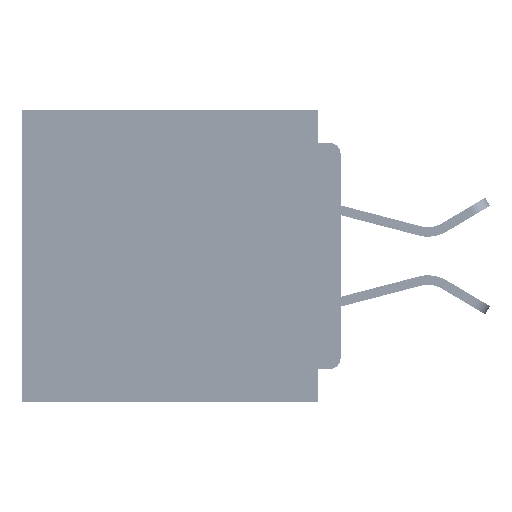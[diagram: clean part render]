
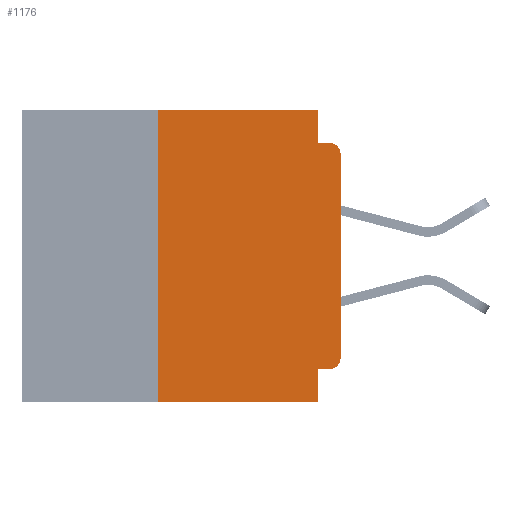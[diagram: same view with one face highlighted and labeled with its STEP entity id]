
A CAD part, left-side view. The second image highlights one B-rep face of the part: STEP entity #1176.
In plain terms, the highlighted planar face has unit normal (-1, 0, 0).
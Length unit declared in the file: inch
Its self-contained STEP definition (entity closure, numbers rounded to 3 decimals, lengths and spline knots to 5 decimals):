
#187 = LINE ( 'NONE', #39883, #10791 ) ;
#500 = CIRCLE ( 'NONE', #19951, 0.015 ) ;
#1176 = ADVANCED_FACE ( 'NONE', ( #3654 ), #41799, .F. ) ;
#2094 = CARTESIAN_POINT ( 'NONE',  ( 0., 0.25, -0.4 ) ) ;
#2684 = CARTESIAN_POINT ( 'NONE',  ( 0., 0.031, 0. ) ) ;
#3654 = FACE_OUTER_BOUND ( 'NONE', #29090, .T. ) ;
#3697 = VECTOR ( 'NONE', #33979, 39.37008 ) ;
#4495 = VECTOR ( 'NONE', #24936, 39.37008 ) ;
#5057 = EDGE_CURVE ( 'NONE', #32782, #6862, #44740, .T. ) ;
#5749 = ORIENTED_EDGE ( 'NONE', *, *, #19472, .T. ) ;
#6282 = DIRECTION ( 'NONE',  ( 0., -1., 0. ) ) ;
#6862 = VERTEX_POINT ( 'NONE', #33075 ) ;
#7333 = ORIENTED_EDGE ( 'NONE', *, *, #5057, .F. ) ;
#7449 = DIRECTION ( 'NONE',  ( -1., 0., 0. ) ) ;
#9366 = EDGE_CURVE ( 'NONE', #20051, #9809, #41578, .T. ) ;
#9436 = LINE ( 'NONE', #13655, #43655 ) ;
#9809 = VERTEX_POINT ( 'NONE', #24323 ) ;
#10075 = CARTESIAN_POINT ( 'NONE',  ( 0., 0.031, -0.355 ) ) ;
#10219 = CIRCLE ( 'NONE', #50465, 0.015 ) ;
#10791 = VECTOR ( 'NONE', #44306, 39.37008 ) ;
#13051 = VERTEX_POINT ( 'NONE', #51636 ) ;
#13473 = VERTEX_POINT ( 'NONE', #10075 ) ;
#13654 = VECTOR ( 'NONE', #21131, 39.37008 ) ;
#13655 = CARTESIAN_POINT ( 'NONE',  ( 0., 0., -0.355 ) ) ;
#14047 = LINE ( 'NONE', #21825, #36419 ) ;
#15650 = LINE ( 'NONE', #2684, #3697 ) ;
#15993 = ORIENTED_EDGE ( 'NONE', *, *, #42915, .T. ) ;
#16497 = CARTESIAN_POINT ( 'NONE',  ( 0., 0.031, -0.4 ) ) ;
#19472 = EDGE_CURVE ( 'NONE', #13051, #6862, #10219, .T. ) ;
#19951 = AXIS2_PLACEMENT_3D ( 'NONE', #26772, #50992, #31278 ) ;
#20051 = VERTEX_POINT ( 'NONE', #42547 ) ;
#21131 = DIRECTION ( 'NONE',  ( 0., 0., -1. ) ) ;
#21825 = CARTESIAN_POINT ( 'NONE',  ( 0., 0.437, -0.4 ) ) ;
#21854 = EDGE_CURVE ( 'NONE', #9809, #32782, #15650, .T. ) ;
#23982 = EDGE_CURVE ( 'NONE', #43362, #13051, #56915, .T. ) ;
#24014 = DIRECTION ( 'NONE',  ( 0., 0., -1. ) ) ;
#24038 = DIRECTION ( 'NONE',  ( 0., 0., 1. ) ) ;
#24323 = CARTESIAN_POINT ( 'NONE',  ( 0., 0.031, 0. ) ) ;
#24450 = EDGE_CURVE ( 'NONE', #47695, #13473, #9436, .T. ) ;
#24936 = DIRECTION ( 'NONE',  ( 0., -1., 0. ) ) ;
#25518 = ORIENTED_EDGE ( 'NONE', *, *, #21854, .F. ) ;
#26325 = DIRECTION ( 'NONE',  ( 0., -1., 0. ) ) ;
#26772 = CARTESIAN_POINT ( 'NONE',  ( 0., 0.015, -0.34 ) ) ;
#26990 = AXIS2_PLACEMENT_3D ( 'NONE', #46237, #50698, #24014 ) ;
#29090 = EDGE_LOOP ( 'NONE', ( #35580, #5749, #7333, #25518, #45500, #33915, #36617, #45672, #42423, #15993 ) ) ;
#31278 = DIRECTION ( 'NONE',  ( 0., 0., -1. ) ) ;
#31662 = EDGE_CURVE ( 'NONE', #13473, #36514, #49212, .T. ) ;
#32782 = VERTEX_POINT ( 'NONE', #33944 ) ;
#33075 = CARTESIAN_POINT ( 'NONE',  ( 0., 0.015, -0.045 ) ) ;
#33915 = ORIENTED_EDGE ( 'NONE', *, *, #48504, .F. ) ;
#33944 = CARTESIAN_POINT ( 'NONE',  ( 0., 0.031, -0.045 ) ) ;
#33979 = DIRECTION ( 'NONE',  ( 0., 0., -1. ) ) ;
#34220 = CARTESIAN_POINT ( 'NONE',  ( 0., 0.015, -0.06 ) ) ;
#35580 = ORIENTED_EDGE ( 'NONE', *, *, #23982, .T. ) ;
#35932 = DIRECTION ( 'NONE',  ( 0., 1., 0. ) ) ;
#36419 = VECTOR ( 'NONE', #26325, 39.37008 ) ;
#36514 = VERTEX_POINT ( 'NONE', #57645 ) ;
#36617 = ORIENTED_EDGE ( 'NONE', *, *, #54879, .T. ) ;
#38745 = DIRECTION ( 'NONE',  ( 0., 0., -1. ) ) ;
#39883 = CARTESIAN_POINT ( 'NONE',  ( 0., 0.25, -0.4 ) ) ;
#41477 = CARTESIAN_POINT ( 'NONE',  ( 0., 0.015, -0.355 ) ) ;
#41578 = LINE ( 'NONE', #42890, #4495 ) ;
#41799 = PLANE ( 'NONE',  #26990 ) ;
#41821 = CARTESIAN_POINT ( 'NONE',  ( 0., 0., 0. ) ) ;
#42423 = ORIENTED_EDGE ( 'NONE', *, *, #24450, .F. ) ;
#42547 = CARTESIAN_POINT ( 'NONE',  ( 0., 0.25, 0. ) ) ;
#42890 = CARTESIAN_POINT ( 'NONE',  ( 0., 0.437, 0. ) ) ;
#42915 = EDGE_CURVE ( 'NONE', #47695, #43362, #500, .T. ) ;
#43139 = CARTESIAN_POINT ( 'NONE',  ( 0., 0., -0.34 ) ) ;
#43362 = VERTEX_POINT ( 'NONE', #43139 ) ;
#43655 = VECTOR ( 'NONE', #35932, 39.37008 ) ;
#44306 = DIRECTION ( 'NONE',  ( 0., 0., 1. ) ) ;
#44740 = LINE ( 'NONE', #46481, #56569 ) ;
#45081 = VECTOR ( 'NONE', #24038, 39.37008 ) ;
#45500 = ORIENTED_EDGE ( 'NONE', *, *, #9366, .F. ) ;
#45672 = ORIENTED_EDGE ( 'NONE', *, *, #31662, .F. ) ;
#46237 = CARTESIAN_POINT ( 'NONE',  ( 0., 0.437, 0. ) ) ;
#46481 = CARTESIAN_POINT ( 'NONE',  ( 0., 0., -0.045 ) ) ;
#47695 = VERTEX_POINT ( 'NONE', #41477 ) ;
#48504 = EDGE_CURVE ( 'NONE', #50664, #20051, #187, .T. ) ;
#49212 = LINE ( 'NONE', #16497, #13654 ) ;
#50465 = AXIS2_PLACEMENT_3D ( 'NONE', #34220, #7449, #38745 ) ;
#50664 = VERTEX_POINT ( 'NONE', #2094 ) ;
#50698 = DIRECTION ( 'NONE',  ( 1., 0., 0. ) ) ;
#50992 = DIRECTION ( 'NONE',  ( -1., 0., 0. ) ) ;
#51636 = CARTESIAN_POINT ( 'NONE',  ( 0., 0., -0.06 ) ) ;
#54879 = EDGE_CURVE ( 'NONE', #50664, #36514, #14047, .T. ) ;
#56569 = VECTOR ( 'NONE', #6282, 39.37008 ) ;
#56915 = LINE ( 'NONE', #41821, #45081 ) ;
#57645 = CARTESIAN_POINT ( 'NONE',  ( 0., 0.031, -0.4 ) ) ;
